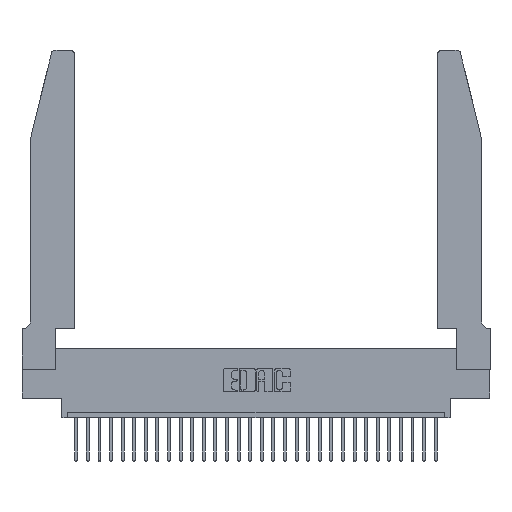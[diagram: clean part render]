
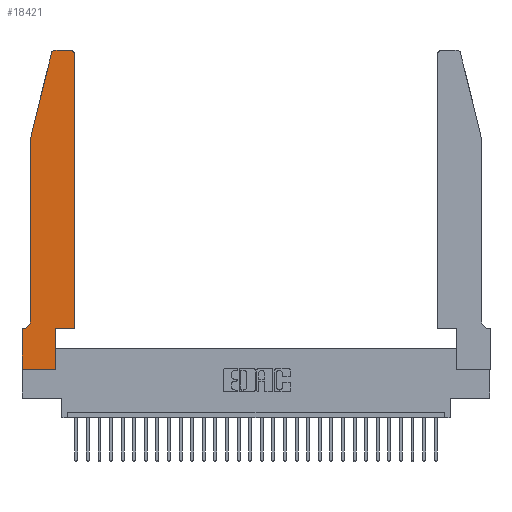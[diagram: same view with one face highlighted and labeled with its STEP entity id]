
A CAD part, top view. The second image highlights one B-rep face of the part: STEP entity #18421.
In plain terms, the highlighted planar face has unit normal (0, 0, 1).
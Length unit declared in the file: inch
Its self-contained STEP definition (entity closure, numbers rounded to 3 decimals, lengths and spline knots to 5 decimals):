
#404 = ORIENTED_EDGE ( 'NONE', *, *, #1506, .T. ) ;
#1397 = ORIENTED_EDGE ( 'NONE', *, *, #28257, .T. ) ;
#1455 = VERTEX_POINT ( 'NONE', #2216 ) ;
#1506 = EDGE_CURVE ( 'NONE', #20908, #22361, #10397, .T. ) ;
#1510 = VERTEX_POINT ( 'NONE', #14248 ) ;
#1554 = DIRECTION ( 'NONE',  ( 0., 0., 1. ) ) ;
#2022 = CARTESIAN_POINT ( 'NONE',  ( 0., 0.35, 0.37 ) ) ;
#2116 = CARTESIAN_POINT ( 'NONE',  ( 0.0755, 0.42, 0.37 ) ) ;
#2216 = CARTESIAN_POINT ( 'NONE',  ( 0.4505, 2.72, 0.37 ) ) ;
#2746 = EDGE_CURVE ( 'NONE', #1510, #8276, #15445, .T. ) ;
#2830 = CARTESIAN_POINT ( 'NONE',  ( 0.0055, 0.35, 0.37 ) ) ;
#3013 = AXIS2_PLACEMENT_3D ( 'NONE', #25899, #11833, #26108 ) ;
#3503 = PLANE ( 'NONE',  #13195 ) ;
#3587 = VECTOR ( 'NONE', #9222, 39.37008 ) ;
#3903 = CARTESIAN_POINT ( 'NONE',  ( 0.284, 2.75, 0.37 ) ) ;
#3907 = VERTEX_POINT ( 'NONE', #27752 ) ;
#3962 = DIRECTION ( 'NONE',  ( 0., -1., 0. ) ) ;
#4108 = VECTOR ( 'NONE', #14146, 39.37008 ) ;
#4337 = CARTESIAN_POINT ( 'NONE',  ( 0.0755, 2., 0.37 ) ) ;
#4380 = ORIENTED_EDGE ( 'NONE', *, *, #23058, .T. ) ;
#5111 = EDGE_LOOP ( 'NONE', ( #25187, #24573, #24115, #25207, #1397, #14939, #4380, #404, #14704, #18890, #30356, #5934 ) ) ;
#5934 = ORIENTED_EDGE ( 'NONE', *, *, #11984, .T. ) ;
#6079 = EDGE_CURVE ( 'NONE', #14268, #1455, #22670, .T. ) ;
#7450 = CARTESIAN_POINT ( 'NONE',  ( 0.284, 2.72, 0.37 ) ) ;
#7831 = VERTEX_POINT ( 'NONE', #24456 ) ;
#8259 = CIRCLE ( 'NONE', #3013, 0.07 ) ;
#8276 = VERTEX_POINT ( 'NONE', #23635 ) ;
#8550 = CARTESIAN_POINT ( 'NONE',  ( 0.4505, 0.35, 0.37 ) ) ;
#9185 = LINE ( 'NONE', #16261, #20526 ) ;
#9222 = DIRECTION ( 'NONE',  ( 0., 1., 0. ) ) ;
#10397 = LINE ( 'NONE', #27748, #25811 ) ;
#10565 = CARTESIAN_POINT ( 'NONE',  ( 0.2865, 0., 0.37 ) ) ;
#10606 = LINE ( 'NONE', #23901, #19470 ) ;
#10841 = VECTOR ( 'NONE', #22317, 39.37008 ) ;
#10916 = CIRCLE ( 'NONE', #26225, 0.03 ) ;
#11130 = CARTESIAN_POINT ( 'NONE',  ( 0.4505, 0.35, 0.37 ) ) ;
#11415 = DIRECTION ( 'NONE',  ( 1., 0., 0. ) ) ;
#11559 = LINE ( 'NONE', #12681, #10841 ) ;
#11833 = DIRECTION ( 'NONE',  ( 0., 0., -1. ) ) ;
#11984 = EDGE_CURVE ( 'NONE', #1455, #3907, #26446, .T. ) ;
#12681 = CARTESIAN_POINT ( 'NONE',  ( 0.0755, 2., 0.37 ) ) ;
#13129 = DIRECTION ( 'NONE',  ( 0., 0., 1. ) ) ;
#13195 = AXIS2_PLACEMENT_3D ( 'NONE', #29233, #1554, #15316 ) ;
#14146 = DIRECTION ( 'NONE',  ( 1., 0., 0. ) ) ;
#14248 = CARTESIAN_POINT ( 'NONE',  ( 0.25487, 2.72718, 0.37 ) ) ;
#14268 = VERTEX_POINT ( 'NONE', #11130 ) ;
#14704 = ORIENTED_EDGE ( 'NONE', *, *, #20574, .T. ) ;
#14939 = ORIENTED_EDGE ( 'NONE', *, *, #18068, .T. ) ;
#15316 = DIRECTION ( 'NONE',  ( 1., 0., 0. ) ) ;
#15445 = LINE ( 'NONE', #4337, #26539 ) ;
#16116 = CARTESIAN_POINT ( 'NONE',  ( 0., 0., 0.37 ) ) ;
#16261 = CARTESIAN_POINT ( 'NONE',  ( 0.0755, 0.35, 0.37 ) ) ;
#17637 = LINE ( 'NONE', #27162, #23912 ) ;
#18068 = EDGE_CURVE ( 'NONE', #28181, #29601, #9185, .T. ) ;
#18421 = ADVANCED_FACE ( 'NONE', ( #27165 ), #3503, .T. ) ;
#18484 = CARTESIAN_POINT ( 'NONE',  ( 0.2865, 0.35, 0.37 ) ) ;
#18890 = ORIENTED_EDGE ( 'NONE', *, *, #23337, .T. ) ;
#19470 = VECTOR ( 'NONE', #21414, 39.37008 ) ;
#19547 = EDGE_CURVE ( 'NONE', #22393, #1510, #10916, .T. ) ;
#19991 = CARTESIAN_POINT ( 'NONE',  ( 0.4205, 2.72, 0.37 ) ) ;
#20324 = DIRECTION ( 'NONE',  ( -0.239, -0.971, 0. ) ) ;
#20400 = AXIS2_PLACEMENT_3D ( 'NONE', #19991, #13129, #29654 ) ;
#20526 = VECTOR ( 'NONE', #25447, 39.37008 ) ;
#20574 = EDGE_CURVE ( 'NONE', #22361, #7831, #22997, .T. ) ;
#20908 = VERTEX_POINT ( 'NONE', #16116 ) ;
#21339 = VERTEX_POINT ( 'NONE', #2116 ) ;
#21414 = DIRECTION ( 'NONE',  ( -1., 0., 0. ) ) ;
#21512 = VECTOR ( 'NONE', #24963, 39.37008 ) ;
#22317 = DIRECTION ( 'NONE',  ( 0., -1., 0. ) ) ;
#22361 = VERTEX_POINT ( 'NONE', #10565 ) ;
#22393 = VERTEX_POINT ( 'NONE', #3903 ) ;
#22670 = LINE ( 'NONE', #8550, #21512 ) ;
#22997 = LINE ( 'NONE', #18484, #3587 ) ;
#23058 = EDGE_CURVE ( 'NONE', #29601, #20908, #17637, .T. ) ;
#23337 = EDGE_CURVE ( 'NONE', #7831, #14268, #25758, .T. ) ;
#23635 = CARTESIAN_POINT ( 'NONE',  ( 0.0755, 2., 0.37 ) ) ;
#23715 = CARTESIAN_POINT ( 'NONE',  ( 0.4505, 0.35, 0.37 ) ) ;
#23901 = CARTESIAN_POINT ( 'NONE',  ( 0.2605, 2.75, 0.37 ) ) ;
#23909 = DIRECTION ( 'NONE',  ( 1., 0., 0. ) ) ;
#23912 = VECTOR ( 'NONE', #3962, 39.37008 ) ;
#24115 = ORIENTED_EDGE ( 'NONE', *, *, #2746, .T. ) ;
#24456 = CARTESIAN_POINT ( 'NONE',  ( 0.2865, 0.35, 0.37 ) ) ;
#24573 = ORIENTED_EDGE ( 'NONE', *, *, #19547, .T. ) ;
#24963 = DIRECTION ( 'NONE',  ( 0., 1., 0. ) ) ;
#25187 = ORIENTED_EDGE ( 'NONE', *, *, #30299, .T. ) ;
#25207 = ORIENTED_EDGE ( 'NONE', *, *, #27841, .T. ) ;
#25447 = DIRECTION ( 'NONE',  ( -1., 0., 0. ) ) ;
#25758 = LINE ( 'NONE', #23715, #4108 ) ;
#25811 = VECTOR ( 'NONE', #11415, 39.37008 ) ;
#25899 = CARTESIAN_POINT ( 'NONE',  ( 0.0055, 0.42, 0.37 ) ) ;
#26108 = DIRECTION ( 'NONE',  ( -1., 0., 0. ) ) ;
#26225 = AXIS2_PLACEMENT_3D ( 'NONE', #7450, #28558, #23909 ) ;
#26446 = CIRCLE ( 'NONE', #20400, 0.03 ) ;
#26539 = VECTOR ( 'NONE', #20324, 39.37008 ) ;
#27162 = CARTESIAN_POINT ( 'NONE',  ( 0., 0., 0.37 ) ) ;
#27165 = FACE_OUTER_BOUND ( 'NONE', #5111, .T. ) ;
#27748 = CARTESIAN_POINT ( 'NONE',  ( 0., 0., 0.37 ) ) ;
#27752 = CARTESIAN_POINT ( 'NONE',  ( 0.4205, 2.75, 0.37 ) ) ;
#27841 = EDGE_CURVE ( 'NONE', #8276, #21339, #11559, .T. ) ;
#28181 = VERTEX_POINT ( 'NONE', #2830 ) ;
#28257 = EDGE_CURVE ( 'NONE', #21339, #28181, #8259, .T. ) ;
#28558 = DIRECTION ( 'NONE',  ( 0., 0., 1. ) ) ;
#29233 = CARTESIAN_POINT ( 'NONE',  ( 0., 0.35, 0.37 ) ) ;
#29601 = VERTEX_POINT ( 'NONE', #2022 ) ;
#29654 = DIRECTION ( 'NONE',  ( 1., 0., 0. ) ) ;
#30299 = EDGE_CURVE ( 'NONE', #3907, #22393, #10606, .T. ) ;
#30356 = ORIENTED_EDGE ( 'NONE', *, *, #6079, .T. ) ;
